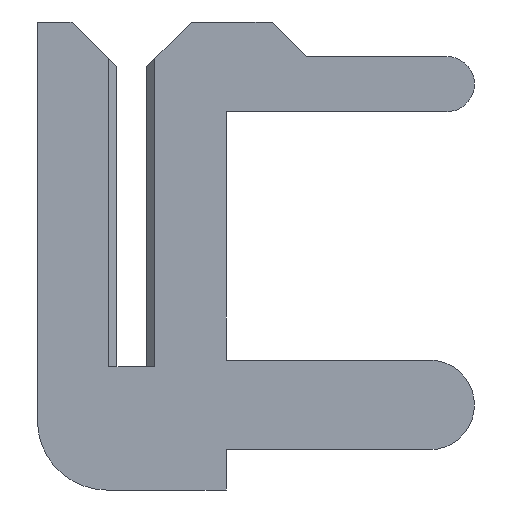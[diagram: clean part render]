
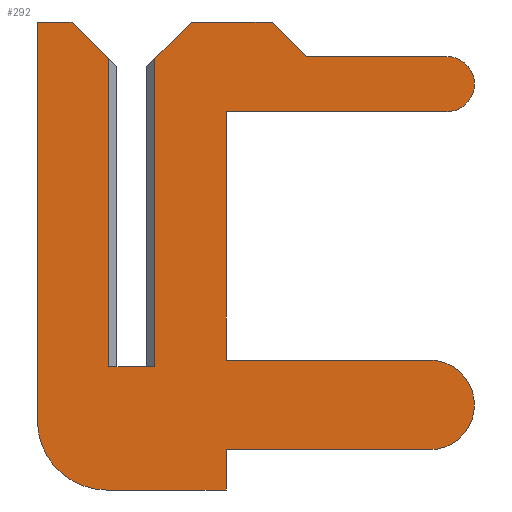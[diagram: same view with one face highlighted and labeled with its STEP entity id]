
A CAD part, left-side view. The second image highlights one B-rep face of the part: STEP entity #292.
In plain terms, the highlighted planar face has unit normal (-1, 0, 0).
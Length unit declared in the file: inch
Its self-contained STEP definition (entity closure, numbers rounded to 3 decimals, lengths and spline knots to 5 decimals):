
#18 = DIRECTION ( 'NONE',  ( 0., 0., 1. ) ) ;
#19 = DIRECTION ( 'NONE',  ( 0., 0., -1. ) ) ;
#32 = DIRECTION ( 'NONE',  ( 0., -0.707, -0.707 ) ) ;
#34 = CIRCLE ( 'NONE', #565, 0.03 ) ;
#38 = ORIENTED_EDGE ( 'NONE', *, *, #374, .F. ) ;
#42 = ORIENTED_EDGE ( 'NONE', *, *, #588, .F. ) ;
#49 = DIRECTION ( 'NONE',  ( 0., 0., -1. ) ) ;
#51 = LINE ( 'NONE', #387, #988 ) ;
#60 = LINE ( 'NONE', #627, #580 ) ;
#67 = ORIENTED_EDGE ( 'NONE', *, *, #156, .F. ) ;
#77 = CARTESIAN_POINT ( 'NONE',  ( -0.01, 0.011, -0.0535 ) ) ;
#80 = EDGE_CURVE ( 'NONE', #421, #1163, #131, .T. ) ;
#91 = CIRCLE ( 'NONE', #404, 0.0195 ) ;
#95 = CARTESIAN_POINT ( 'NONE',  ( -0.01, -0.1295, -0.0165 ) ) ;
#96 = ORIENTED_EDGE ( 'NONE', *, *, #910, .F. ) ;
#108 = DIRECTION ( 'NONE',  ( 0., -1., 0. ) ) ;
#131 = LINE ( 'NONE', #366, #532 ) ;
#139 = LINE ( 'NONE', #503, #961 ) ;
#146 = VERTEX_POINT ( 'NONE', #975 ) ;
#151 = LINE ( 'NONE', #959, #663 ) ;
#155 = ORIENTED_EDGE ( 'NONE', *, *, #795, .F. ) ;
#156 = EDGE_CURVE ( 'NONE', #995, #195, #34, .T. ) ;
#176 = LINE ( 'NONE', #842, #371 ) ;
#179 = CARTESIAN_POINT ( 'NONE',  ( -0.01, 0.041, -0.0235 ) ) ;
#195 = VERTEX_POINT ( 'NONE', #179 ) ;
#205 = LINE ( 'NONE', #330, #1155 ) ;
#212 = CARTESIAN_POINT ( 'NONE',  ( -0.01, 0.026, 0.15 ) ) ;
#222 = CARTESIAN_POINT ( 'NONE',  ( -0.01, -0.1295, 0.003 ) ) ;
#228 = VERTEX_POINT ( 'NONE', #990 ) ;
#233 = LINE ( 'NONE', #308, #693 ) ;
#236 = CIRCLE ( 'NONE', #1093, 0.012 ) ;
#245 = DIRECTION ( 'NONE',  ( 0., -0.707, -0.707 ) ) ;
#246 = VERTEX_POINT ( 'NONE', #287 ) ;
#253 = CARTESIAN_POINT ( 'NONE',  ( -0.01, -0.041, 0.111 ) ) ;
#267 = ORIENTED_EDGE ( 'NONE', *, *, #611, .F. ) ;
#277 = PLANE ( 'NONE',  #867 ) ;
#283 = VECTOR ( 'NONE', #303, 39.37008 ) ;
#287 = CARTESIAN_POINT ( 'NONE',  ( -0.01, 0.01, 0.134 ) ) ;
#292 = ADVANCED_FACE ( 'NONE', ( #442 ), #277, .T. ) ;
#293 = VERTEX_POINT ( 'NONE', #468 ) ;
#303 = DIRECTION ( 'NONE',  ( 0., -1., 0. ) ) ;
#308 = CARTESIAN_POINT ( 'NONE',  ( -0.01, -0.026, 0.15 ) ) ;
#325 = CARTESIAN_POINT ( 'NONE',  ( -0.01, -0.01, 0.134 ) ) ;
#328 = CARTESIAN_POINT ( 'NONE',  ( -0.01, -0.01, 0. ) ) ;
#330 = CARTESIAN_POINT ( 'NONE',  ( -0.01, -0.076, 0.135 ) ) ;
#331 = ORIENTED_EDGE ( 'NONE', *, *, #792, .F. ) ;
#353 = VERTEX_POINT ( 'NONE', #212 ) ;
#357 = CARTESIAN_POINT ( 'NONE',  ( -0.01, -0.137, 0.135 ) ) ;
#363 = VECTOR ( 'NONE', #1109, 39.37008 ) ;
#365 = EDGE_CURVE ( 'NONE', #1031, #353, #609, .T. ) ;
#366 = CARTESIAN_POINT ( 'NONE',  ( -0.01, -0.0065, 0.1305 ) ) ;
#371 = VECTOR ( 'NONE', #19, 39.37008 ) ;
#374 = EDGE_CURVE ( 'NONE', #630, #515, #176, .T. ) ;
#387 = CARTESIAN_POINT ( 'NONE',  ( -0.01, -0.041, 0.111 ) ) ;
#404 = AXIS2_PLACEMENT_3D ( 'NONE', #95, #574, #18 ) ;
#408 = ORIENTED_EDGE ( 'NONE', *, *, #1098, .F. ) ;
#421 = VERTEX_POINT ( 'NONE', #325 ) ;
#424 = ORIENTED_EDGE ( 'NONE', *, *, #365, .F. ) ;
#431 = LINE ( 'NONE', #77, #720 ) ;
#442 = FACE_OUTER_BOUND ( 'NONE', #964, .T. ) ;
#447 = LINE ( 'NONE', #866, #571 ) ;
#465 = LINE ( 'NONE', #923, #363 ) ;
#466 = CARTESIAN_POINT ( 'NONE',  ( -0.01, -0.1295, 0.003 ) ) ;
#468 = CARTESIAN_POINT ( 'NONE',  ( -0.01, -0.061, 0.15 ) ) ;
#471 = CARTESIAN_POINT ( 'NONE',  ( -0.01, -0.041, 0.003 ) ) ;
#503 = CARTESIAN_POINT ( 'NONE',  ( -0.01, 0.01, -0.0235 ) ) ;
#515 = VERTEX_POINT ( 'NONE', #952 ) ;
#528 = DIRECTION ( 'NONE',  ( 0., -1., 0. ) ) ;
#532 = VECTOR ( 'NONE', #710, 39.37008 ) ;
#560 = LINE ( 'NONE', #1170, #946 ) ;
#565 = AXIS2_PLACEMENT_3D ( 'NONE', #636, #736, #820 ) ;
#571 = VECTOR ( 'NONE', #49, 39.37008 ) ;
#574 = DIRECTION ( 'NONE',  ( 1., 0., 0. ) ) ;
#580 = VECTOR ( 'NONE', #970, 39.37008 ) ;
#583 = DIRECTION ( 'NONE',  ( 0., 0., 1. ) ) ;
#588 = EDGE_CURVE ( 'NONE', #293, #228, #205, .T. ) ;
#589 = VERTEX_POINT ( 'NONE', #1046 ) ;
#603 = ORIENTED_EDGE ( 'NONE', *, *, #999, .F. ) ;
#609 = LINE ( 'NONE', #765, #1125 ) ;
#611 = EDGE_CURVE ( 'NONE', #1163, #293, #233, .T. ) ;
#627 = CARTESIAN_POINT ( 'NONE',  ( -0.01, -0.01, 0.15 ) ) ;
#628 = VECTOR ( 'NONE', #1143, 39.37008 ) ;
#630 = VERTEX_POINT ( 'NONE', #746 ) ;
#636 = CARTESIAN_POINT ( 'NONE',  ( -0.01, 0.011, -0.0235 ) ) ;
#637 = EDGE_CURVE ( 'NONE', #840, #630, #984, .T. ) ;
#644 = CARTESIAN_POINT ( 'NONE',  ( -0.01, -0.041, -0.036 ) ) ;
#648 = DIRECTION ( 'NONE',  ( 0., 1., 0. ) ) ;
#650 = DIRECTION ( 'NONE',  ( 0., -1., 0. ) ) ;
#663 = VECTOR ( 'NONE', #245, 39.37008 ) ;
#684 = EDGE_CURVE ( 'NONE', #589, #881, #1039, .T. ) ;
#688 = DIRECTION ( 'NONE',  ( 0., 0., 1. ) ) ;
#693 = VECTOR ( 'NONE', #650, 39.37008 ) ;
#694 = VECTOR ( 'NONE', #1026, 39.37008 ) ;
#695 = CARTESIAN_POINT ( 'NONE',  ( -0.01, -0.137, 0.123 ) ) ;
#710 = DIRECTION ( 'NONE',  ( 0., -0.707, 0.707 ) ) ;
#720 = VECTOR ( 'NONE', #892, 39.37008 ) ;
#727 = VERTEX_POINT ( 'NONE', #466 ) ;
#736 = DIRECTION ( 'NONE',  ( 1., 0., 0. ) ) ;
#737 = DIRECTION ( 'NONE',  ( 0., 0., 1. ) ) ;
#740 = ORIENTED_EDGE ( 'NONE', *, *, #80, .F. ) ;
#746 = CARTESIAN_POINT ( 'NONE',  ( -0.01, -0.041, -0.036 ) ) ;
#765 = CARTESIAN_POINT ( 'NONE',  ( -0.01, 0.026, 0.15 ) ) ;
#766 = EDGE_CURVE ( 'NONE', #195, #1031, #465, .T. ) ;
#770 = CARTESIAN_POINT ( 'NONE',  ( -0.01, -0.1295, -0.036 ) ) ;
#784 = CARTESIAN_POINT ( 'NONE',  ( -0.01, 0.011, -0.0535 ) ) ;
#792 = EDGE_CURVE ( 'NONE', #727, #840, #91, .T. ) ;
#795 = EDGE_CURVE ( 'NONE', #146, #1117, #51, .T. ) ;
#808 = ORIENTED_EDGE ( 'NONE', *, *, #766, .F. ) ;
#810 = ORIENTED_EDGE ( 'NONE', *, *, #1129, .T. ) ;
#820 = DIRECTION ( 'NONE',  ( 0., 0., 1. ) ) ;
#822 = VERTEX_POINT ( 'NONE', #471 ) ;
#836 = CARTESIAN_POINT ( 'NONE',  ( -0.01, 0.0065, 0. ) ) ;
#840 = VERTEX_POINT ( 'NONE', #770 ) ;
#842 = CARTESIAN_POINT ( 'NONE',  ( -0.01, -0.041, -0.0535 ) ) ;
#852 = EDGE_CURVE ( 'NONE', #822, #727, #1113, .T. ) ;
#865 = EDGE_CURVE ( 'NONE', #589, #246, #139, .T. ) ;
#866 = CARTESIAN_POINT ( 'NONE',  ( -0.01, -0.041, 0.003 ) ) ;
#867 = AXIS2_PLACEMENT_3D ( 'NONE', #902, #1105, #737 ) ;
#881 = VERTEX_POINT ( 'NONE', #328 ) ;
#892 = DIRECTION ( 'NONE',  ( 0., 1., 0. ) ) ;
#902 = CARTESIAN_POINT ( 'NONE',  ( -0.01, 0.011, -0.0235 ) ) ;
#910 = EDGE_CURVE ( 'NONE', #1117, #822, #447, .T. ) ;
#923 = CARTESIAN_POINT ( 'NONE',  ( -0.01, 0.041, 0.15 ) ) ;
#925 = ORIENTED_EDGE ( 'NONE', *, *, #1116, .F. ) ;
#946 = VECTOR ( 'NONE', #528, 39.37008 ) ;
#952 = CARTESIAN_POINT ( 'NONE',  ( -0.01, -0.041, -0.0535 ) ) ;
#959 = CARTESIAN_POINT ( 'NONE',  ( -0.01, 0.0065, 0.1305 ) ) ;
#961 = VECTOR ( 'NONE', #583, 39.37008 ) ;
#964 = EDGE_LOOP ( 'NONE', ( #740, #810, #1057, #1147, #603, #424, #808, #67, #408, #38, #1101, #331, #1088, #96, #155, #1115, #925, #42, #267 ) ) ;
#968 = EDGE_CURVE ( 'NONE', #1190, #146, #236, .T. ) ;
#970 = DIRECTION ( 'NONE',  ( 0., 0., -1. ) ) ;
#975 = CARTESIAN_POINT ( 'NONE',  ( -0.01, -0.137, 0.111 ) ) ;
#984 = LINE ( 'NONE', #644, #694 ) ;
#988 = VECTOR ( 'NONE', #648, 39.37008 ) ;
#990 = CARTESIAN_POINT ( 'NONE',  ( -0.01, -0.076, 0.135 ) ) ;
#995 = VERTEX_POINT ( 'NONE', #784 ) ;
#999 = EDGE_CURVE ( 'NONE', #353, #246, #151, .T. ) ;
#1026 = DIRECTION ( 'NONE',  ( 0., 1., 0. ) ) ;
#1031 = VERTEX_POINT ( 'NONE', #1161 ) ;
#1039 = LINE ( 'NONE', #836, #283 ) ;
#1046 = CARTESIAN_POINT ( 'NONE',  ( -0.01, 0.01, 0. ) ) ;
#1057 = ORIENTED_EDGE ( 'NONE', *, *, #684, .F. ) ;
#1081 = CARTESIAN_POINT ( 'NONE',  ( -0.01, -0.026, 0.15 ) ) ;
#1088 = ORIENTED_EDGE ( 'NONE', *, *, #852, .F. ) ;
#1093 = AXIS2_PLACEMENT_3D ( 'NONE', #695, #1157, #688 ) ;
#1098 = EDGE_CURVE ( 'NONE', #515, #995, #431, .T. ) ;
#1101 = ORIENTED_EDGE ( 'NONE', *, *, #637, .F. ) ;
#1105 = DIRECTION ( 'NONE',  ( -1., 0., 0. ) ) ;
#1109 = DIRECTION ( 'NONE',  ( 0., 0., 1. ) ) ;
#1113 = LINE ( 'NONE', #222, #628 ) ;
#1115 = ORIENTED_EDGE ( 'NONE', *, *, #968, .F. ) ;
#1116 = EDGE_CURVE ( 'NONE', #228, #1190, #560, .T. ) ;
#1117 = VERTEX_POINT ( 'NONE', #253 ) ;
#1125 = VECTOR ( 'NONE', #108, 39.37008 ) ;
#1129 = EDGE_CURVE ( 'NONE', #421, #881, #60, .T. ) ;
#1143 = DIRECTION ( 'NONE',  ( 0., -1., 0. ) ) ;
#1147 = ORIENTED_EDGE ( 'NONE', *, *, #865, .T. ) ;
#1155 = VECTOR ( 'NONE', #32, 39.37008 ) ;
#1157 = DIRECTION ( 'NONE',  ( 1., 0., 0. ) ) ;
#1161 = CARTESIAN_POINT ( 'NONE',  ( -0.01, 0.041, 0.15 ) ) ;
#1163 = VERTEX_POINT ( 'NONE', #1081 ) ;
#1170 = CARTESIAN_POINT ( 'NONE',  ( -0.01, -0.137, 0.135 ) ) ;
#1190 = VERTEX_POINT ( 'NONE', #357 ) ;
